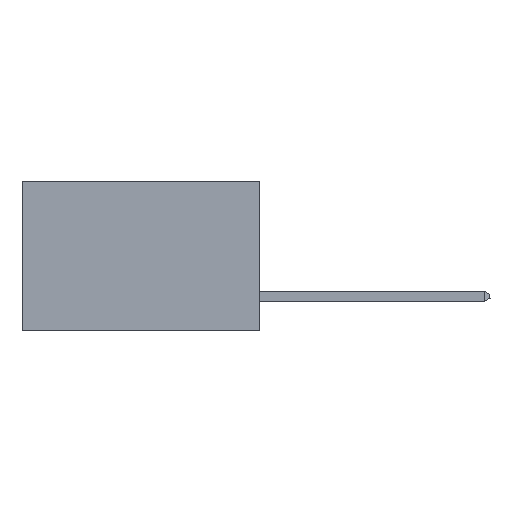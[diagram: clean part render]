
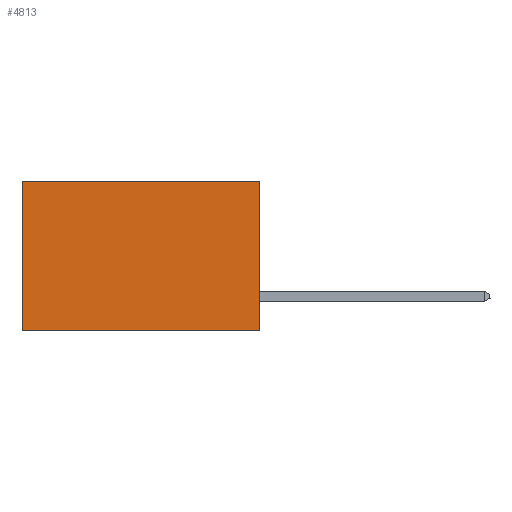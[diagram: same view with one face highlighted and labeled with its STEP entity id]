
A CAD part, left-side view. The second image highlights one B-rep face of the part: STEP entity #4813.
In plain terms, the highlighted planar face has unit normal (-1, 0, 0).
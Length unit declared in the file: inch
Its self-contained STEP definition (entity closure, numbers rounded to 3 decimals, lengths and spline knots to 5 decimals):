
#1330 = CARTESIAN_POINT ( 'NONE',  ( 0.277, 0.59, -0.37 ) ) ;
#4057 = LINE ( 'NONE', #26977, #4722 ) ;
#4142 = VERTEX_POINT ( 'NONE', #1330 ) ;
#4722 = VECTOR ( 'NONE', #26731, 39.37008 ) ;
#4813 = ADVANCED_FACE ( 'NONE', ( #26928 ), #18363, .F. ) ;
#5219 = DIRECTION ( 'NONE',  ( 0., 0., -1. ) ) ;
#5487 = EDGE_CURVE ( 'NONE', #9408, #4142, #4057, .T. ) ;
#6066 = CARTESIAN_POINT ( 'NONE',  ( 0.277, 0.59, 0. ) ) ;
#6854 = VECTOR ( 'NONE', #14649, 39.37008 ) ;
#7710 = VECTOR ( 'NONE', #18808, 39.37008 ) ;
#8429 = ORIENTED_EDGE ( 'NONE', *, *, #27963, .F. ) ;
#9067 = VERTEX_POINT ( 'NONE', #15894 ) ;
#9132 = EDGE_LOOP ( 'NONE', ( #18286, #8429, #11533, #19884 ) ) ;
#9408 = VERTEX_POINT ( 'NONE', #6066 ) ;
#11533 = ORIENTED_EDGE ( 'NONE', *, *, #15486, .F. ) ;
#12647 = LINE ( 'NONE', #25395, #6854 ) ;
#14649 = DIRECTION ( 'NONE',  ( 0., 1., 0. ) ) ;
#14819 = VERTEX_POINT ( 'NONE', #24882 ) ;
#15340 = VECTOR ( 'NONE', #5219, 39.37008 ) ;
#15486 = EDGE_CURVE ( 'NONE', #14819, #9067, #21101, .T. ) ;
#15894 = CARTESIAN_POINT ( 'NONE',  ( 0.277, 0., -0.37 ) ) ;
#16654 = CARTESIAN_POINT ( 'NONE',  ( 0.277, 0., -0.37 ) ) ;
#18039 = DIRECTION ( 'NONE',  ( 0., 0., -1. ) ) ;
#18156 = DIRECTION ( 'NONE',  ( 1., 0., 0. ) ) ;
#18286 = ORIENTED_EDGE ( 'NONE', *, *, #5487, .T. ) ;
#18313 = CARTESIAN_POINT ( 'NONE',  ( 0.277, 0., -0.37 ) ) ;
#18363 = PLANE ( 'NONE',  #21850 ) ;
#18808 = DIRECTION ( 'NONE',  ( 0., 1., 0. ) ) ;
#19884 = ORIENTED_EDGE ( 'NONE', *, *, #26455, .T. ) ;
#21101 = LINE ( 'NONE', #26835, #15340 ) ;
#21850 = AXIS2_PLACEMENT_3D ( 'NONE', #18313, #18156, #18039 ) ;
#24882 = CARTESIAN_POINT ( 'NONE',  ( 0.277, 0., 0. ) ) ;
#25088 = LINE ( 'NONE', #16654, #7710 ) ;
#25395 = CARTESIAN_POINT ( 'NONE',  ( 0.277, 0., 0. ) ) ;
#26455 = EDGE_CURVE ( 'NONE', #14819, #9408, #12647, .T. ) ;
#26731 = DIRECTION ( 'NONE',  ( 0., 0., -1. ) ) ;
#26835 = CARTESIAN_POINT ( 'NONE',  ( 0.277, 0., -0.37 ) ) ;
#26928 = FACE_OUTER_BOUND ( 'NONE', #9132, .T. ) ;
#26977 = CARTESIAN_POINT ( 'NONE',  ( 0.277, 0.59, -0.37 ) ) ;
#27963 = EDGE_CURVE ( 'NONE', #9067, #4142, #25088, .T. ) ;
